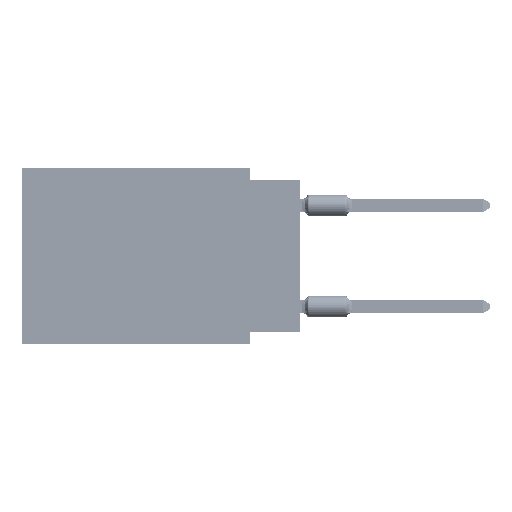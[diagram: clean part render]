
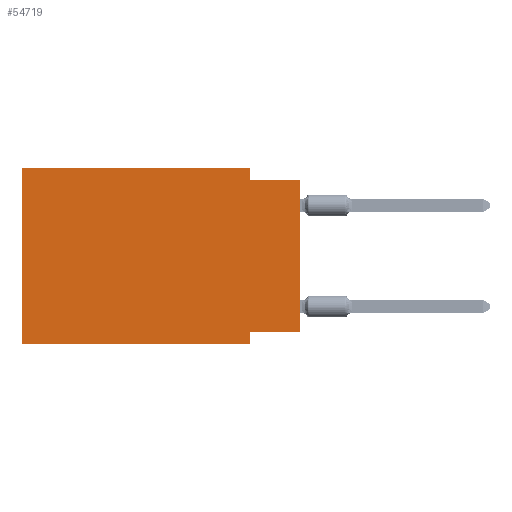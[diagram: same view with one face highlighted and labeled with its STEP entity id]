
A CAD part, left-side view. The second image highlights one B-rep face of the part: STEP entity #54719.
In plain terms, the highlighted planar face has unit normal (-1, 0, 0).
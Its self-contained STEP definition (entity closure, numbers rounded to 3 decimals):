
#1132 = CARTESIAN_POINT ( 'NONE',  ( 0., 2.54, 0. ) ) ;
#2139 = CARTESIAN_POINT ( 'NONE',  ( 0., 13.97, -8.89 ) ) ;
#3554 = CARTESIAN_POINT ( 'NONE',  ( 0., 2.54, -8.89 ) ) ;
#5316 = FACE_OUTER_BOUND ( 'NONE', #88170, .T. ) ;
#5664 = ORIENTED_EDGE ( 'NONE', *, *, #63806, .F. ) ;
#6746 = CARTESIAN_POINT ( 'NONE',  ( 0., 0., -8.255 ) ) ;
#7939 = DIRECTION ( 'NONE',  ( 0., -1., 0. ) ) ;
#8655 = DIRECTION ( 'NONE',  ( 0., 0., -1. ) ) ;
#9378 = ORIENTED_EDGE ( 'NONE', *, *, #10608, .F. ) ;
#10608 = EDGE_CURVE ( 'NONE', #35626, #13729, #101754, .T. ) ;
#11440 = EDGE_CURVE ( 'NONE', #64312, #20285, #18349, .T. ) ;
#12722 = EDGE_CURVE ( 'NONE', #13729, #64312, #63409, .T. ) ;
#13729 = VERTEX_POINT ( 'NONE', #98463 ) ;
#15600 = EDGE_CURVE ( 'NONE', #93440, #43271, #32351, .T. ) ;
#18349 = LINE ( 'NONE', #1132, #53123 ) ;
#18452 = VECTOR ( 'NONE', #41198, 1000. ) ;
#19569 = VECTOR ( 'NONE', #39130, 1000. ) ;
#20053 = ORIENTED_EDGE ( 'NONE', *, *, #44262, .F. ) ;
#20285 = VERTEX_POINT ( 'NONE', #54307 ) ;
#23119 = CARTESIAN_POINT ( 'NONE',  ( 0., 13.97, -8.89 ) ) ;
#24735 = CARTESIAN_POINT ( 'NONE',  ( 0., 2.54, 0. ) ) ;
#27163 = VERTEX_POINT ( 'NONE', #3554 ) ;
#27556 = VECTOR ( 'NONE', #96744, 1000. ) ;
#28878 = AXIS2_PLACEMENT_3D ( 'NONE', #92968, #63212, #46020 ) ;
#31602 = DIRECTION ( 'NONE',  ( 0., -1., 0. ) ) ;
#32351 = LINE ( 'NONE', #65711, #18452 ) ;
#33589 = EDGE_CURVE ( 'NONE', #35626, #27163, #96644, .T. ) ;
#33713 = LINE ( 'NONE', #40507, #47841 ) ;
#35626 = VERTEX_POINT ( 'NONE', #2139 ) ;
#36322 = ORIENTED_EDGE ( 'NONE', *, *, #46143, .F. ) ;
#38599 = DIRECTION ( 'NONE',  ( 0., 1., 0. ) ) ;
#39130 = DIRECTION ( 'NONE',  ( 0., 0., 1. ) ) ;
#40507 = CARTESIAN_POINT ( 'NONE',  ( 0., 2.54, -8.89 ) ) ;
#41198 = DIRECTION ( 'NONE',  ( 0., 0., 1. ) ) ;
#43271 = VERTEX_POINT ( 'NONE', #46447 ) ;
#44262 = EDGE_CURVE ( 'NONE', #20285, #43271, #64933, .T. ) ;
#45597 = VERTEX_POINT ( 'NONE', #50329 ) ;
#45947 = VECTOR ( 'NONE', #7939, 1000. ) ;
#46020 = DIRECTION ( 'NONE',  ( 0., 0., -1. ) ) ;
#46143 = EDGE_CURVE ( 'NONE', #93440, #45597, #86057, .T. ) ;
#46447 = CARTESIAN_POINT ( 'NONE',  ( 0., 0., -0.635 ) ) ;
#46456 = CARTESIAN_POINT ( 'NONE',  ( 0., 13.97, 0. ) ) ;
#47751 = CARTESIAN_POINT ( 'NONE',  ( 0., 13.97, 0. ) ) ;
#47841 = VECTOR ( 'NONE', #8655, 1000. ) ;
#50329 = CARTESIAN_POINT ( 'NONE',  ( 0., 2.54, -8.255 ) ) ;
#53123 = VECTOR ( 'NONE', #80481, 1000. ) ;
#54307 = CARTESIAN_POINT ( 'NONE',  ( 0., 2.54, -0.635 ) ) ;
#54719 = ADVANCED_FACE ( 'NONE', ( #5316 ), #86694, .F. ) ;
#61503 = ORIENTED_EDGE ( 'NONE', *, *, #15600, .T. ) ;
#62745 = ORIENTED_EDGE ( 'NONE', *, *, #33589, .T. ) ;
#63212 = DIRECTION ( 'NONE',  ( 1., 0., 0. ) ) ;
#63409 = LINE ( 'NONE', #47751, #96362 ) ;
#63806 = EDGE_CURVE ( 'NONE', #45597, #27163, #33713, .T. ) ;
#64312 = VERTEX_POINT ( 'NONE', #24735 ) ;
#64933 = LINE ( 'NONE', #81092, #27556 ) ;
#65711 = CARTESIAN_POINT ( 'NONE',  ( 0., 0., 0. ) ) ;
#71255 = ORIENTED_EDGE ( 'NONE', *, *, #12722, .F. ) ;
#80481 = DIRECTION ( 'NONE',  ( 0., 0., -1. ) ) ;
#81092 = CARTESIAN_POINT ( 'NONE',  ( 0., 0., -0.635 ) ) ;
#86057 = LINE ( 'NONE', #6746, #87860 ) ;
#86694 = PLANE ( 'NONE',  #28878 ) ;
#87847 = ORIENTED_EDGE ( 'NONE', *, *, #11440, .F. ) ;
#87860 = VECTOR ( 'NONE', #38599, 1000. ) ;
#88170 = EDGE_LOOP ( 'NONE', ( #61503, #20053, #87847, #71255, #9378, #62745, #5664, #36322 ) ) ;
#92968 = CARTESIAN_POINT ( 'NONE',  ( 0., 13.97, 0. ) ) ;
#93440 = VERTEX_POINT ( 'NONE', #99367 ) ;
#96362 = VECTOR ( 'NONE', #31602, 1000. ) ;
#96644 = LINE ( 'NONE', #23119, #45947 ) ;
#96744 = DIRECTION ( 'NONE',  ( 0., -1., 0. ) ) ;
#98463 = CARTESIAN_POINT ( 'NONE',  ( 0., 13.97, 0. ) ) ;
#99367 = CARTESIAN_POINT ( 'NONE',  ( 0., 0., -8.255 ) ) ;
#101754 = LINE ( 'NONE', #46456, #19569 ) ;
